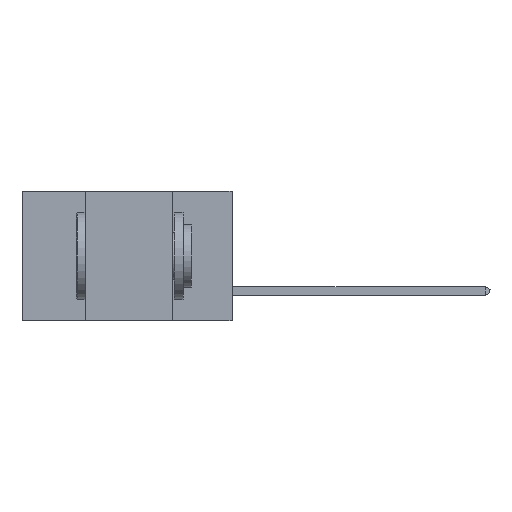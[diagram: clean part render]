
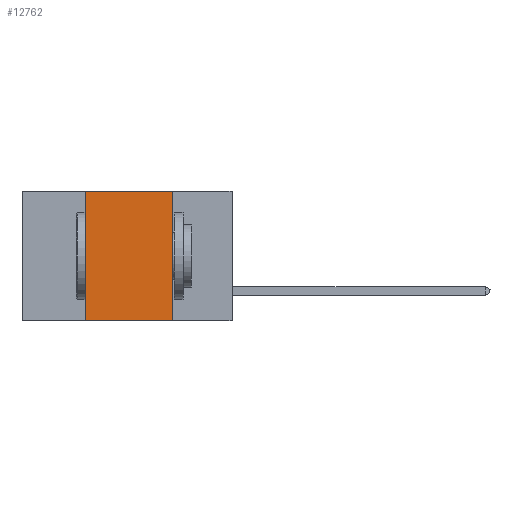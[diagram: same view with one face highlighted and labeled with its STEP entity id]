
A CAD part, left-side view. The second image highlights one B-rep face of the part: STEP entity #12762.
In plain terms, the highlighted planar face has unit normal (-1, 0, 0).
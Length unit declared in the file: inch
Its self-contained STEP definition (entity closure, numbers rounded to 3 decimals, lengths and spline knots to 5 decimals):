
#196 = DIRECTION ( 'NONE',  ( 0., 0., -1. ) ) ;
#768 = VECTOR ( 'NONE', #12275, 39.37008 ) ;
#910 = ORIENTED_EDGE ( 'NONE', *, *, #13385, .F. ) ;
#1664 = ORIENTED_EDGE ( 'NONE', *, *, #8059, .F. ) ;
#1718 = LINE ( 'NONE', #8432, #11564 ) ;
#3529 = DIRECTION ( 'NONE',  ( 0., -1., 0. ) ) ;
#4187 = PLANE ( 'NONE',  #10762 ) ;
#4892 = ORIENTED_EDGE ( 'NONE', *, *, #12496, .T. ) ;
#5734 = DIRECTION ( 'NONE',  ( 1., 0., 0. ) ) ;
#5750 = ORIENTED_EDGE ( 'NONE', *, *, #5875, .F. ) ;
#5875 = EDGE_CURVE ( 'NONE', #16638, #8894, #16197, .T. ) ;
#6868 = VERTEX_POINT ( 'NONE', #16863 ) ;
#8059 = EDGE_CURVE ( 'NONE', #6868, #16638, #12013, .T. ) ;
#8432 = CARTESIAN_POINT ( 'NONE',  ( 0., 0.6, -0.37 ) ) ;
#8657 = CARTESIAN_POINT ( 'NONE',  ( 0., 0.17, 0. ) ) ;
#8894 = VERTEX_POINT ( 'NONE', #17815 ) ;
#10725 = CARTESIAN_POINT ( 'NONE',  ( 0., 0.42, 0. ) ) ;
#10762 = AXIS2_PLACEMENT_3D ( 'NONE', #12053, #5734, #196 ) ;
#10771 = LINE ( 'NONE', #8657, #18960 ) ;
#10850 = EDGE_LOOP ( 'NONE', ( #910, #5750, #1664, #4892 ) ) ;
#11564 = VECTOR ( 'NONE', #11614, 39.37008 ) ;
#11588 = VERTEX_POINT ( 'NONE', #16451 ) ;
#11614 = DIRECTION ( 'NONE',  ( 0., -1., 0. ) ) ;
#12013 = LINE ( 'NONE', #10725, #768 ) ;
#12053 = CARTESIAN_POINT ( 'NONE',  ( 0., 0.6, 0. ) ) ;
#12089 = VECTOR ( 'NONE', #3529, 39.37008 ) ;
#12242 = CARTESIAN_POINT ( 'NONE',  ( 0., 0.42, 0. ) ) ;
#12275 = DIRECTION ( 'NONE',  ( 0., 0., 1. ) ) ;
#12496 = EDGE_CURVE ( 'NONE', #6868, #11588, #1718, .T. ) ;
#12762 = ADVANCED_FACE ( 'NONE', ( #13682 ), #4187, .F. ) ;
#13385 = EDGE_CURVE ( 'NONE', #8894, #11588, #10771, .T. ) ;
#13682 = FACE_OUTER_BOUND ( 'NONE', #10850, .T. ) ;
#16197 = LINE ( 'NONE', #16454, #12089 ) ;
#16451 = CARTESIAN_POINT ( 'NONE',  ( 0., 0.17, -0.37 ) ) ;
#16454 = CARTESIAN_POINT ( 'NONE',  ( 0., 0.6, 0. ) ) ;
#16638 = VERTEX_POINT ( 'NONE', #12242 ) ;
#16863 = CARTESIAN_POINT ( 'NONE',  ( 0., 0.42, -0.37 ) ) ;
#17815 = CARTESIAN_POINT ( 'NONE',  ( 0., 0.17, 0. ) ) ;
#18960 = VECTOR ( 'NONE', #19400, 39.37008 ) ;
#19400 = DIRECTION ( 'NONE',  ( 0., 0., -1. ) ) ;
